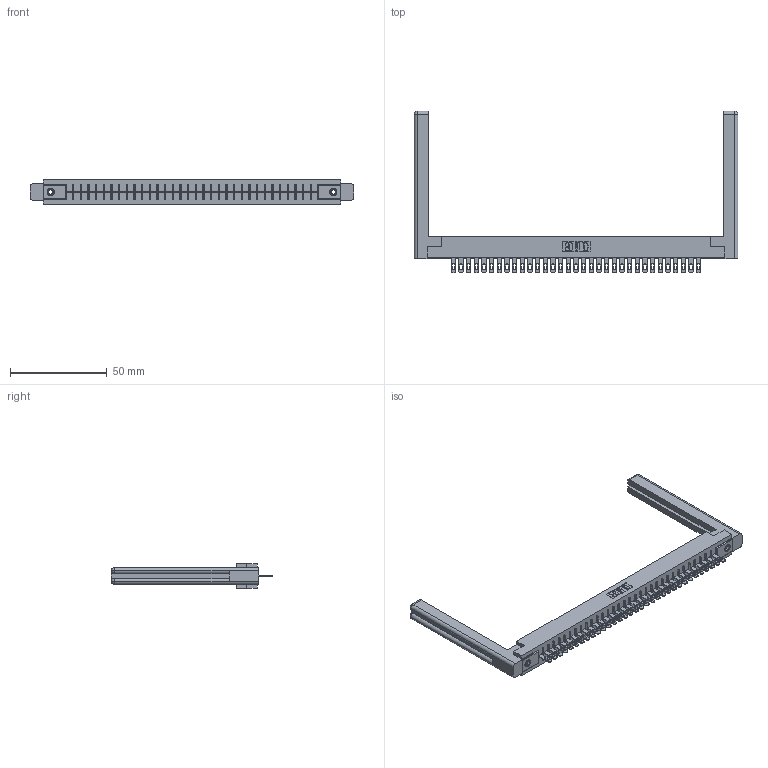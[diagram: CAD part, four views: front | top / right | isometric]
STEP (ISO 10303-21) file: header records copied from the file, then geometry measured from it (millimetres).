
FILE_DESCRIPTION (( 'STEP AP203' ), '1' );
FILE_NAME ('356-033-500-158.STEP', '2018-08-01T21:22:32', ( '' ), ( '' ), 'SwSTEP 2.0', 'SolidWorks 2016', '' );
FILE_SCHEMA (( 'CONFIG_CONTROL_DESIGN' ));
Length unit declared in the file: inch
Products named in the file (5): 306-290-001_100; 345-250-001_345-250-001-102; 307-220-058; 356-033-500-158; 306 Part_.156 Dia
Assembly tree (38 placements, depth 2):
  356-033-500-158
    306 Part_.156 Dia
    306-290-001_100  x33
    345-250-001_345-250-001-102  x2
    307-220-058  x2
Bounding box: 167.39 x 83.52 x 12.7 mm (x, y, z)
Volume: 25604.5 mm3; surface area: 24633.6 mm2
Topology: 38 solids, 38 shells, 2766 faces, 7765 edges, 4986 vertices
Faces by surface type: plane 1802, cylinder 808, sphere 132, cone 12, torus 12
Entity records: 34737 total; most frequent: CARTESIAN_POINT 5841, ORIENTED_EDGE 5732, DIRECTION 5716, EDGE_CURVE 2866, VECTOR 2230, LINE 2230, VERTEX_POINT 1814, AXIS2_PLACEMENT_3D 1743
